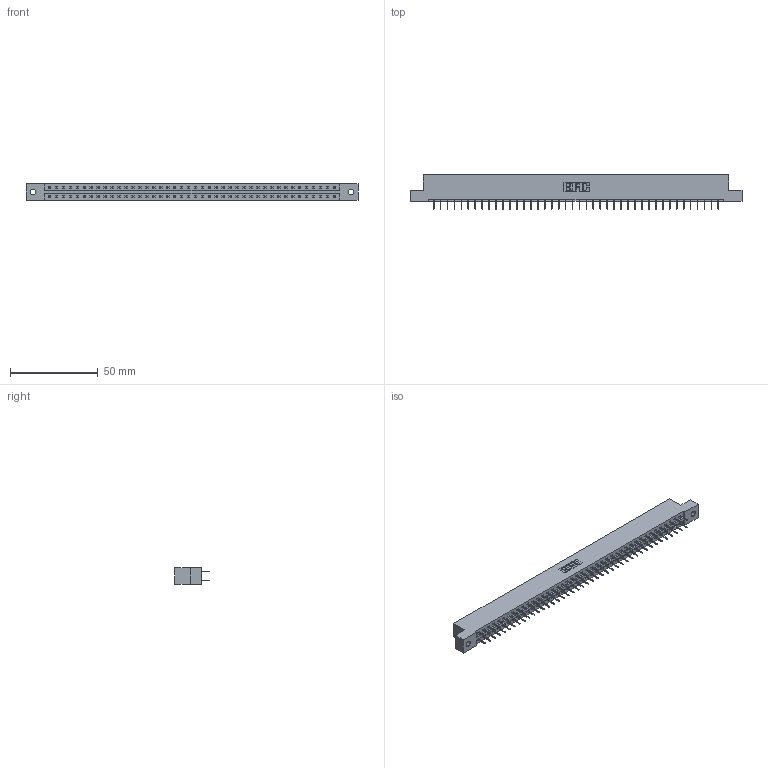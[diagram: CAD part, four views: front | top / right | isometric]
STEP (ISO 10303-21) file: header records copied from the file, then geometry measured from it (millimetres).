
FILE_DESCRIPTION (( 'STEP AP203' ), '1' );
FILE_NAME ('337-084-524-202.STEP', '2019-10-10T13:52:29', ( '' ), ( '' ), 'SwSTEP 2.0', 'SolidWorks 2016', '' );
FILE_SCHEMA (( 'CONFIG_CONTROL_DESIGN' ));
Length unit declared in the file: inch
Products named in the file (3): 337-084-524-202; 345-292-001_345-293-124; 337 Part_Flush Mounting Lugs - 0.128 Dia
Assembly tree (85 placements, depth 2):
  337-084-524-202
    337 Part_Flush Mounting Lugs - 0.128 Dia
    345-292-001_345-293-124  x84
Bounding box: 189.43 x 19.69 x 9.4 mm (x, y, z)
Volume: 19800.2 mm3; surface area: 21717.7 mm2
Topology: 85 solids, 85 shells, 4986 faces, 14171 edges, 9110 vertices
Faces by surface type: plane 3766, cylinder 1220
Entity records: 32641 total; most frequent: CARTESIAN_POINT 5498, ORIENTED_EDGE 5434, DIRECTION 4677, EDGE_CURVE 2717, LINE 2593, VECTOR 2593, VERTEX_POINT 1806, AXIS2_PLACEMENT_3D 1042
